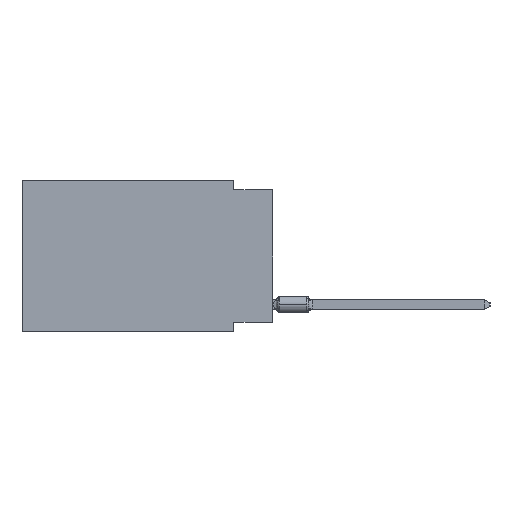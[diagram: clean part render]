
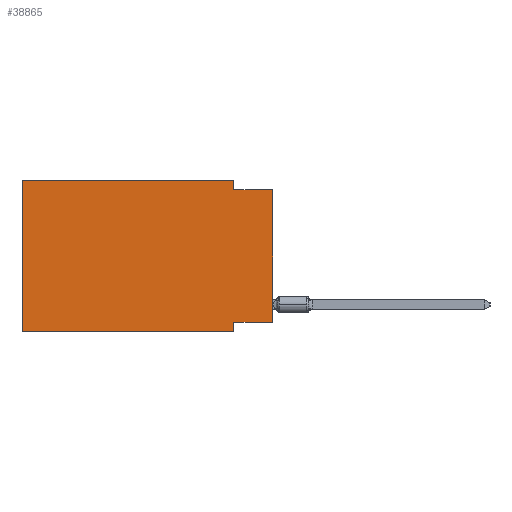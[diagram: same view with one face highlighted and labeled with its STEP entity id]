
A CAD part, left-side view. The second image highlights one B-rep face of the part: STEP entity #38865.
In plain terms, the highlighted planar face has unit normal (-1, 0, 0).
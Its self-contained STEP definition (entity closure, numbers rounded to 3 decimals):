
#1289 = CARTESIAN_POINT ( 'NONE',  ( 0., 16.383, -9.906 ) ) ;
#1437 = VERTEX_POINT ( 'NONE', #30796 ) ;
#1601 = VECTOR ( 'NONE', #34349, 1000. ) ;
#2891 = VECTOR ( 'NONE', #7243, 1000. ) ;
#4599 = CARTESIAN_POINT ( 'NONE',  ( 0., 2.54, -0.635 ) ) ;
#4663 = EDGE_CURVE ( 'NONE', #24503, #38813, #41230, .T. ) ;
#6322 = EDGE_CURVE ( 'NONE', #18061, #9268, #23330, .T. ) ;
#7243 = DIRECTION ( 'NONE',  ( 0., 0., -1. ) ) ;
#8593 = VECTOR ( 'NONE', #46300, 1000. ) ;
#8682 = CARTESIAN_POINT ( 'NONE',  ( 0., 16.383, 0. ) ) ;
#9241 = VECTOR ( 'NONE', #22100, 1000. ) ;
#9268 = VERTEX_POINT ( 'NONE', #24125 ) ;
#9319 = EDGE_LOOP ( 'NONE', ( #16190, #13127, #36747, #45431, #19085, #10224, #31303, #27349 ) ) ;
#10224 = ORIENTED_EDGE ( 'NONE', *, *, #4663, .T. ) ;
#13127 = ORIENTED_EDGE ( 'NONE', *, *, #17057, .F. ) ;
#13163 = VECTOR ( 'NONE', #27365, 1000. ) ;
#13814 = DIRECTION ( 'NONE',  ( 0., 0., 1. ) ) ;
#14033 = PLANE ( 'NONE',  #44693 ) ;
#14143 = CARTESIAN_POINT ( 'NONE',  ( 0., 0., -9.271 ) ) ;
#14263 = EDGE_CURVE ( 'NONE', #24503, #32153, #43025, .T. ) ;
#14975 = CARTESIAN_POINT ( 'NONE',  ( 0., 2.54, 0. ) ) ;
#16190 = ORIENTED_EDGE ( 'NONE', *, *, #28683, .T. ) ;
#17057 = EDGE_CURVE ( 'NONE', #37016, #1437, #29055, .T. ) ;
#17630 = CARTESIAN_POINT ( 'NONE',  ( 0., 0., -0.635 ) ) ;
#18061 = VERTEX_POINT ( 'NONE', #14143 ) ;
#19085 = ORIENTED_EDGE ( 'NONE', *, *, #14263, .F. ) ;
#22100 = DIRECTION ( 'NONE',  ( 0., 0., -1. ) ) ;
#23330 = LINE ( 'NONE', #45186, #13163 ) ;
#24125 = CARTESIAN_POINT ( 'NONE',  ( 0., 2.54, -9.271 ) ) ;
#24503 = VERTEX_POINT ( 'NONE', #33153 ) ;
#24851 = CARTESIAN_POINT ( 'NONE',  ( 0., 2.54, 0. ) ) ;
#25004 = CARTESIAN_POINT ( 'NONE',  ( 0., 0., 0. ) ) ;
#26693 = EDGE_CURVE ( 'NONE', #30739, #37016, #39934, .T. ) ;
#27186 = VECTOR ( 'NONE', #31413, 1000. ) ;
#27349 = ORIENTED_EDGE ( 'NONE', *, *, #6322, .F. ) ;
#27365 = DIRECTION ( 'NONE',  ( 0., 1., 0. ) ) ;
#28178 = EDGE_CURVE ( 'NONE', #32153, #30739, #32043, .T. ) ;
#28496 = CARTESIAN_POINT ( 'NONE',  ( 0., 16.383, 0. ) ) ;
#28558 = CARTESIAN_POINT ( 'NONE',  ( 0., 16.383, 0. ) ) ;
#28683 = EDGE_CURVE ( 'NONE', #18061, #1437, #42575, .T. ) ;
#29012 = DIRECTION ( 'NONE',  ( 1., 0., 0. ) ) ;
#29055 = LINE ( 'NONE', #17630, #45838 ) ;
#29262 = DIRECTION ( 'NONE',  ( 0., 0., -1. ) ) ;
#30739 = VERTEX_POINT ( 'NONE', #24851 ) ;
#30796 = CARTESIAN_POINT ( 'NONE',  ( 0., 0., -0.635 ) ) ;
#31303 = ORIENTED_EDGE ( 'NONE', *, *, #40597, .F. ) ;
#31413 = DIRECTION ( 'NONE',  ( 0., 0., 1. ) ) ;
#32043 = LINE ( 'NONE', #28496, #8593 ) ;
#32145 = DIRECTION ( 'NONE',  ( 0., -1., 0. ) ) ;
#32153 = VERTEX_POINT ( 'NONE', #8682 ) ;
#33153 = CARTESIAN_POINT ( 'NONE',  ( 0., 16.383, -9.906 ) ) ;
#34349 = DIRECTION ( 'NONE',  ( 0., -1., 0. ) ) ;
#34972 = CARTESIAN_POINT ( 'NONE',  ( 0., 16.383, 0. ) ) ;
#36373 = CARTESIAN_POINT ( 'NONE',  ( 0., 2.54, -9.906 ) ) ;
#36519 = VECTOR ( 'NONE', #13814, 1000. ) ;
#36742 = LINE ( 'NONE', #43863, #2891 ) ;
#36747 = ORIENTED_EDGE ( 'NONE', *, *, #26693, .F. ) ;
#37016 = VERTEX_POINT ( 'NONE', #4599 ) ;
#38813 = VERTEX_POINT ( 'NONE', #36373 ) ;
#38865 = ADVANCED_FACE ( 'NONE', ( #40177 ), #14033, .F. ) ;
#39934 = LINE ( 'NONE', #14975, #9241 ) ;
#40177 = FACE_OUTER_BOUND ( 'NONE', #9319, .T. ) ;
#40597 = EDGE_CURVE ( 'NONE', #9268, #38813, #36742, .T. ) ;
#41230 = LINE ( 'NONE', #1289, #1601 ) ;
#42575 = LINE ( 'NONE', #25004, #36519 ) ;
#43025 = LINE ( 'NONE', #34972, #27186 ) ;
#43863 = CARTESIAN_POINT ( 'NONE',  ( 0., 2.54, -9.906 ) ) ;
#44693 = AXIS2_PLACEMENT_3D ( 'NONE', #28558, #29012, #29262 ) ;
#45186 = CARTESIAN_POINT ( 'NONE',  ( 0., 0., -9.271 ) ) ;
#45431 = ORIENTED_EDGE ( 'NONE', *, *, #28178, .F. ) ;
#45838 = VECTOR ( 'NONE', #32145, 1000. ) ;
#46300 = DIRECTION ( 'NONE',  ( 0., -1., 0. ) ) ;
